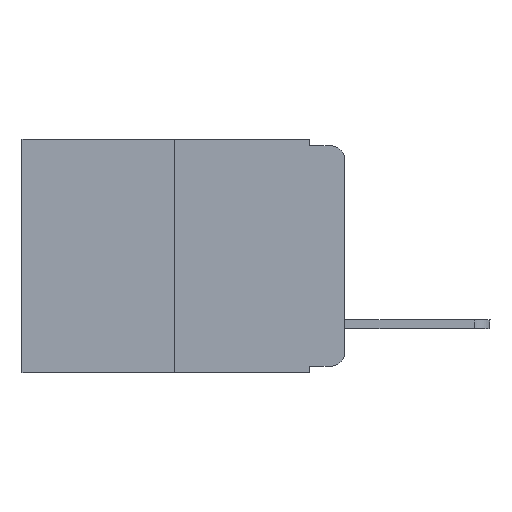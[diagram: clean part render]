
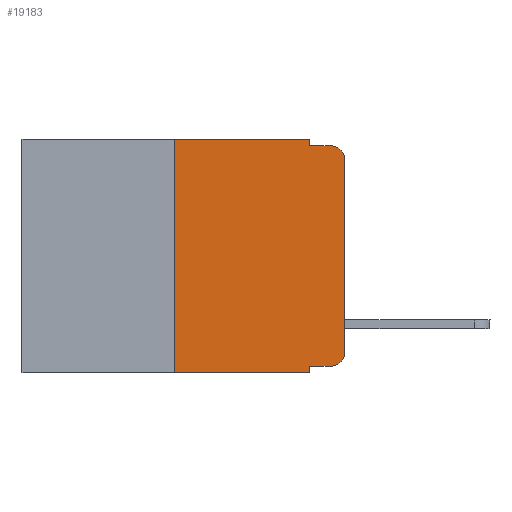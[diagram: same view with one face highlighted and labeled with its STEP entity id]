
A CAD part, left-side view. The second image highlights one B-rep face of the part: STEP entity #19183.
In plain terms, the highlighted planar face has unit normal (-1, 0, 0).
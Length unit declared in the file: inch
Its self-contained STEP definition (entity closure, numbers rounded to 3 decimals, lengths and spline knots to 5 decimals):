
#195 = EDGE_CURVE ( 'NONE', #2741, #16546, #19977, .T. ) ;
#1349 = ORIENTED_EDGE ( 'NONE', *, *, #18034, .T. ) ;
#1850 = VECTOR ( 'NONE', #8230, 39.37008 ) ;
#1923 = LINE ( 'NONE', #13239, #4977 ) ;
#2281 = VERTEX_POINT ( 'NONE', #5447 ) ;
#2526 = VERTEX_POINT ( 'NONE', #12917 ) ;
#2741 = VERTEX_POINT ( 'NONE', #15311 ) ;
#2821 = VERTEX_POINT ( 'NONE', #7593 ) ;
#2916 = CARTESIAN_POINT ( 'NONE',  ( 0., 0.25, 0. ) ) ;
#3661 = LINE ( 'NONE', #19984, #15145 ) ;
#3684 = CARTESIAN_POINT ( 'NONE',  ( 0., 0.051, 0. ) ) ;
#3751 = ORIENTED_EDGE ( 'NONE', *, *, #15179, .T. ) ;
#3896 = EDGE_CURVE ( 'NONE', #9109, #17888, #17099, .T. ) ;
#4200 = ORIENTED_EDGE ( 'NONE', *, *, #19113, .F. ) ;
#4711 = CARTESIAN_POINT ( 'NONE',  ( 0., 0.02, -0.03 ) ) ;
#4899 = VERTEX_POINT ( 'NONE', #14338 ) ;
#4977 = VECTOR ( 'NONE', #16473, 39.37008 ) ;
#5029 = LINE ( 'NONE', #3684, #6266 ) ;
#5389 = CARTESIAN_POINT ( 'NONE',  ( 0., 0.473, -0.343 ) ) ;
#5447 = CARTESIAN_POINT ( 'NONE',  ( 0., 0.051, -0.01 ) ) ;
#5491 = DIRECTION ( 'NONE',  ( 0., -1., 0. ) ) ;
#5597 = LINE ( 'NONE', #19976, #8042 ) ;
#5730 = VERTEX_POINT ( 'NONE', #8323 ) ;
#5734 = ORIENTED_EDGE ( 'NONE', *, *, #195, .T. ) ;
#5903 = DIRECTION ( 'NONE',  ( 1., 0., 0. ) ) ;
#6266 = VECTOR ( 'NONE', #19282, 39.37008 ) ;
#6517 = DIRECTION ( 'NONE',  ( -1., 0., 0. ) ) ;
#6522 = CARTESIAN_POINT ( 'NONE',  ( 0., 0.051, -0.333 ) ) ;
#6901 = VECTOR ( 'NONE', #13065, 39.37008 ) ;
#7470 = CARTESIAN_POINT ( 'NONE',  ( 0., 0.473, 0. ) ) ;
#7593 = CARTESIAN_POINT ( 'NONE',  ( 0., 0.25, 0. ) ) ;
#7612 = ORIENTED_EDGE ( 'NONE', *, *, #15656, .F. ) ;
#7655 = CARTESIAN_POINT ( 'NONE',  ( 0., 0.02, -0.313 ) ) ;
#7778 = DIRECTION ( 'NONE',  ( 0., 0., 1. ) ) ;
#8042 = VECTOR ( 'NONE', #12054, 39.37008 ) ;
#8230 = DIRECTION ( 'NONE',  ( 0., 0., -1. ) ) ;
#8323 = CARTESIAN_POINT ( 'NONE',  ( 0., 0.02, -0.333 ) ) ;
#8502 = CIRCLE ( 'NONE', #15173, 0.02 ) ;
#8592 = CARTESIAN_POINT ( 'NONE',  ( 0., 0.051, 0. ) ) ;
#9109 = VERTEX_POINT ( 'NONE', #14724 ) ;
#9139 = CARTESIAN_POINT ( 'NONE',  ( 0., 0.02, -0.01 ) ) ;
#9406 = DIRECTION ( 'NONE',  ( 0., 0., -1. ) ) ;
#9430 = EDGE_CURVE ( 'NONE', #20058, #2281, #9786, .T. ) ;
#9452 = EDGE_CURVE ( 'NONE', #2821, #20058, #3661, .T. ) ;
#9786 = LINE ( 'NONE', #16143, #1850 ) ;
#10258 = EDGE_CURVE ( 'NONE', #5730, #2526, #8502, .T. ) ;
#10697 = DIRECTION ( 'NONE',  ( 0., 0., -1. ) ) ;
#10779 = AXIS2_PLACEMENT_3D ( 'NONE', #4711, #17313, #9406 ) ;
#11315 = DIRECTION ( 'NONE',  ( 0., 0., -1. ) ) ;
#12054 = DIRECTION ( 'NONE',  ( 0., -1., 0. ) ) ;
#12337 = ORIENTED_EDGE ( 'NONE', *, *, #10258, .T. ) ;
#12917 = CARTESIAN_POINT ( 'NONE',  ( 0., 0., -0.313 ) ) ;
#13065 = DIRECTION ( 'NONE',  ( 0., -1., 0. ) ) ;
#13239 = CARTESIAN_POINT ( 'NONE',  ( 0., 0., 0. ) ) ;
#13416 = ORIENTED_EDGE ( 'NONE', *, *, #13879, .F. ) ;
#13879 = EDGE_CURVE ( 'NONE', #4899, #16546, #5029, .T. ) ;
#14338 = CARTESIAN_POINT ( 'NONE',  ( 0., 0.051, -0.333 ) ) ;
#14677 = VECTOR ( 'NONE', #5491, 39.37008 ) ;
#14724 = CARTESIAN_POINT ( 'NONE',  ( 0., 0., -0.03 ) ) ;
#14918 = VECTOR ( 'NONE', #7778, 39.37008 ) ;
#15145 = VECTOR ( 'NONE', #16542, 39.37008 ) ;
#15173 = AXIS2_PLACEMENT_3D ( 'NONE', #7655, #6517, #11315 ) ;
#15179 = EDGE_CURVE ( 'NONE', #2526, #9109, #1923, .T. ) ;
#15311 = CARTESIAN_POINT ( 'NONE',  ( 0., 0.25, -0.343 ) ) ;
#15529 = ORIENTED_EDGE ( 'NONE', *, *, #9430, .F. ) ;
#15656 = EDGE_CURVE ( 'NONE', #2281, #17888, #5597, .T. ) ;
#15778 = CARTESIAN_POINT ( 'NONE',  ( 0., 0.051, -0.343 ) ) ;
#15916 = PLANE ( 'NONE',  #15936 ) ;
#15936 = AXIS2_PLACEMENT_3D ( 'NONE', #7470, #5903, #10697 ) ;
#16143 = CARTESIAN_POINT ( 'NONE',  ( 0., 0.051, 0. ) ) ;
#16473 = DIRECTION ( 'NONE',  ( 0., 0., 1. ) ) ;
#16542 = DIRECTION ( 'NONE',  ( 0., -1., 0. ) ) ;
#16546 = VERTEX_POINT ( 'NONE', #15778 ) ;
#17099 = CIRCLE ( 'NONE', #10779, 0.02 ) ;
#17151 = LINE ( 'NONE', #2916, #14918 ) ;
#17313 = DIRECTION ( 'NONE',  ( -1., 0., 0. ) ) ;
#17744 = LINE ( 'NONE', #6522, #6901 ) ;
#17888 = VERTEX_POINT ( 'NONE', #9139 ) ;
#18034 = EDGE_CURVE ( 'NONE', #4899, #5730, #17744, .T. ) ;
#18313 = EDGE_LOOP ( 'NONE', ( #3751, #19919, #7612, #15529, #19525, #4200, #5734, #13416, #1349, #12337 ) ) ;
#19113 = EDGE_CURVE ( 'NONE', #2741, #2821, #17151, .T. ) ;
#19183 = ADVANCED_FACE ( 'NONE', ( #20172 ), #15916, .F. ) ;
#19282 = DIRECTION ( 'NONE',  ( 0., 0., -1. ) ) ;
#19525 = ORIENTED_EDGE ( 'NONE', *, *, #9452, .F. ) ;
#19919 = ORIENTED_EDGE ( 'NONE', *, *, #3896, .T. ) ;
#19976 = CARTESIAN_POINT ( 'NONE',  ( 0., 0.051, -0.01 ) ) ;
#19977 = LINE ( 'NONE', #5389, #14677 ) ;
#19984 = CARTESIAN_POINT ( 'NONE',  ( 0., 0.473, 0. ) ) ;
#20058 = VERTEX_POINT ( 'NONE', #8592 ) ;
#20172 = FACE_OUTER_BOUND ( 'NONE', #18313, .T. ) ;
